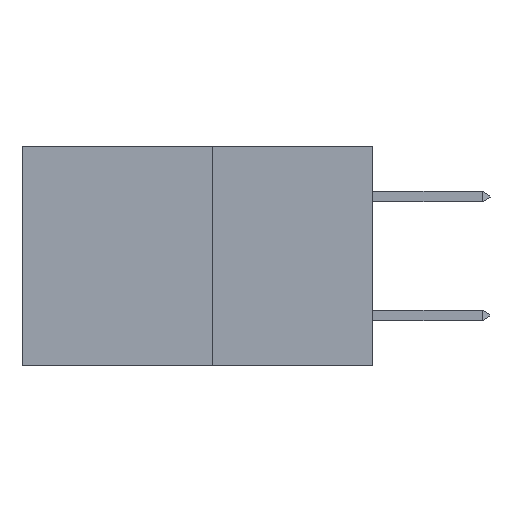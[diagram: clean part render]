
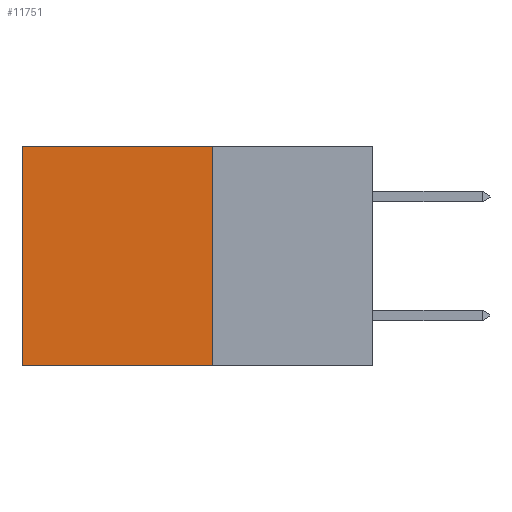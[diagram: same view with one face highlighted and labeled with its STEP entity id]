
A CAD part, left-side view. The second image highlights one B-rep face of the part: STEP entity #11751.
In plain terms, the highlighted planar face has unit normal (-1, 0, 0).
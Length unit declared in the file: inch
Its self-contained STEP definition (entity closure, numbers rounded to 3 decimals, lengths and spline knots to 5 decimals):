
#1081 = PLANE ( 'NONE',  #13051 ) ;
#1846 = DIRECTION ( 'NONE',  ( 0., 1., 0. ) ) ;
#1898 = EDGE_CURVE ( 'NONE', #15765, #15816, #9607, .T. ) ;
#2187 = CARTESIAN_POINT ( 'NONE',  ( 0.277, 0.59, 0. ) ) ;
#2213 = CARTESIAN_POINT ( 'NONE',  ( 0.277, 0.27, -0.37 ) ) ;
#2626 = DIRECTION ( 'NONE',  ( 0., 0., -1. ) ) ;
#2893 = CARTESIAN_POINT ( 'NONE',  ( 0.277, 0.27, 0. ) ) ;
#5186 = DIRECTION ( 'NONE',  ( 0., 0., -1. ) ) ;
#6339 = ORIENTED_EDGE ( 'NONE', *, *, #18374, .F. ) ;
#6761 = DIRECTION ( 'NONE',  ( 0., 0., -1. ) ) ;
#7418 = DIRECTION ( 'NONE',  ( 0., 1., 0. ) ) ;
#7689 = CARTESIAN_POINT ( 'NONE',  ( 0.277, 0.27, 0. ) ) ;
#8634 = VERTEX_POINT ( 'NONE', #2187 ) ;
#9181 = EDGE_LOOP ( 'NONE', ( #16719, #13823, #6339, #16288 ) ) ;
#9607 = LINE ( 'NONE', #16030, #16854 ) ;
#10473 = VECTOR ( 'NONE', #1846, 39.37008 ) ;
#10731 = VECTOR ( 'NONE', #6761, 39.37008 ) ;
#10754 = FACE_OUTER_BOUND ( 'NONE', #9181, .T. ) ;
#11361 = DIRECTION ( 'NONE',  ( 1., 0., 0. ) ) ;
#11751 = ADVANCED_FACE ( 'NONE', ( #10754 ), #1081, .F. ) ;
#12930 = EDGE_CURVE ( 'NONE', #13487, #8634, #14381, .T. ) ;
#13051 = AXIS2_PLACEMENT_3D ( 'NONE', #18501, #11361, #2626 ) ;
#13487 = VERTEX_POINT ( 'NONE', #2893 ) ;
#13823 = ORIENTED_EDGE ( 'NONE', *, *, #1898, .F. ) ;
#14052 = CARTESIAN_POINT ( 'NONE',  ( 0.277, 0.27, -0.37 ) ) ;
#14381 = LINE ( 'NONE', #7689, #10473 ) ;
#14614 = LINE ( 'NONE', #16781, #10731 ) ;
#15739 = EDGE_CURVE ( 'NONE', #8634, #15816, #14614, .T. ) ;
#15765 = VERTEX_POINT ( 'NONE', #14052 ) ;
#15816 = VERTEX_POINT ( 'NONE', #16961 ) ;
#16030 = CARTESIAN_POINT ( 'NONE',  ( 0.277, 0.27, -0.37 ) ) ;
#16098 = LINE ( 'NONE', #2213, #16532 ) ;
#16288 = ORIENTED_EDGE ( 'NONE', *, *, #12930, .T. ) ;
#16532 = VECTOR ( 'NONE', #5186, 39.37008 ) ;
#16719 = ORIENTED_EDGE ( 'NONE', *, *, #15739, .T. ) ;
#16781 = CARTESIAN_POINT ( 'NONE',  ( 0.277, 0.59, -0.37 ) ) ;
#16854 = VECTOR ( 'NONE', #7418, 39.37008 ) ;
#16961 = CARTESIAN_POINT ( 'NONE',  ( 0.277, 0.59, -0.37 ) ) ;
#18374 = EDGE_CURVE ( 'NONE', #13487, #15765, #16098, .T. ) ;
#18501 = CARTESIAN_POINT ( 'NONE',  ( 0.277, 0.27, -0.37 ) ) ;
